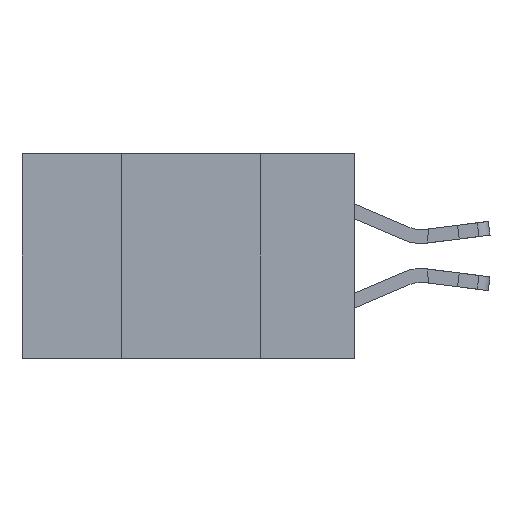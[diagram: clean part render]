
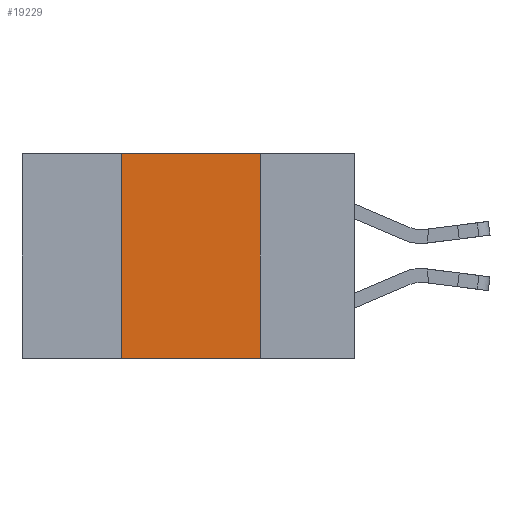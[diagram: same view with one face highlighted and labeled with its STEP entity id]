
A CAD part, left-side view. The second image highlights one B-rep face of the part: STEP entity #19229.
In plain terms, the highlighted planar face has unit normal (-1, 0, 0).
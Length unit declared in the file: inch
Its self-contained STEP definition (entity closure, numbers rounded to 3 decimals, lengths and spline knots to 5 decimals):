
#376 = EDGE_CURVE ( 'NONE', #21886, #20007, #26647, .T. ) ;
#951 = DIRECTION ( 'NONE',  ( 0., -1., 0. ) ) ;
#4375 = ORIENTED_EDGE ( 'NONE', *, *, #23036, .T. ) ;
#5479 = DIRECTION ( 'NONE',  ( 0., -1., 0. ) ) ;
#5638 = PLANE ( 'NONE',  #20766 ) ;
#6726 = VECTOR ( 'NONE', #22529, 39.37008 ) ;
#7437 = ORIENTED_EDGE ( 'NONE', *, *, #376, .F. ) ;
#7907 = DIRECTION ( 'NONE',  ( 1., 0., 0. ) ) ;
#8063 = CARTESIAN_POINT ( 'NONE',  ( 0., 0.42, 0. ) ) ;
#9343 = CARTESIAN_POINT ( 'NONE',  ( 0., 0.17, 0. ) ) ;
#10405 = CARTESIAN_POINT ( 'NONE',  ( 0., 0.17, 0. ) ) ;
#13951 = VECTOR ( 'NONE', #951, 39.37008 ) ;
#14060 = CARTESIAN_POINT ( 'NONE',  ( 0., 0.6, 0. ) ) ;
#15088 = ORIENTED_EDGE ( 'NONE', *, *, #19044, .F. ) ;
#16031 = ORIENTED_EDGE ( 'NONE', *, *, #17144, .F. ) ;
#16291 = CARTESIAN_POINT ( 'NONE',  ( 0., 0.6, -0.37 ) ) ;
#17144 = EDGE_CURVE ( 'NONE', #20007, #23207, #24942, .T. ) ;
#19044 = EDGE_CURVE ( 'NONE', #23207, #25916, #24798, .T. ) ;
#19229 = ADVANCED_FACE ( 'NONE', ( #24440 ), #5638, .F. ) ;
#20007 = VERTEX_POINT ( 'NONE', #23534 ) ;
#20766 = AXIS2_PLACEMENT_3D ( 'NONE', #20992, #7907, #23187 ) ;
#20900 = VECTOR ( 'NONE', #22589, 39.37008 ) ;
#20992 = CARTESIAN_POINT ( 'NONE',  ( 0., 0.6, 0. ) ) ;
#21563 = CARTESIAN_POINT ( 'NONE',  ( 0., 0.42, -0.37 ) ) ;
#21886 = VERTEX_POINT ( 'NONE', #21563 ) ;
#22504 = VECTOR ( 'NONE', #5479, 39.37008 ) ;
#22529 = DIRECTION ( 'NONE',  ( 0., 0., -1. ) ) ;
#22589 = DIRECTION ( 'NONE',  ( 0., 0., 1. ) ) ;
#23036 = EDGE_CURVE ( 'NONE', #21886, #25916, #28276, .T. ) ;
#23187 = DIRECTION ( 'NONE',  ( 0., 0., -1. ) ) ;
#23207 = VERTEX_POINT ( 'NONE', #10405 ) ;
#23273 = CARTESIAN_POINT ( 'NONE',  ( 0., 0.17, -0.37 ) ) ;
#23534 = CARTESIAN_POINT ( 'NONE',  ( 0., 0.42, 0. ) ) ;
#24440 = FACE_OUTER_BOUND ( 'NONE', #27154, .T. ) ;
#24798 = LINE ( 'NONE', #9343, #6726 ) ;
#24942 = LINE ( 'NONE', #14060, #13951 ) ;
#25916 = VERTEX_POINT ( 'NONE', #23273 ) ;
#26647 = LINE ( 'NONE', #8063, #20900 ) ;
#27154 = EDGE_LOOP ( 'NONE', ( #15088, #16031, #7437, #4375 ) ) ;
#28276 = LINE ( 'NONE', #16291, #22504 ) ;
